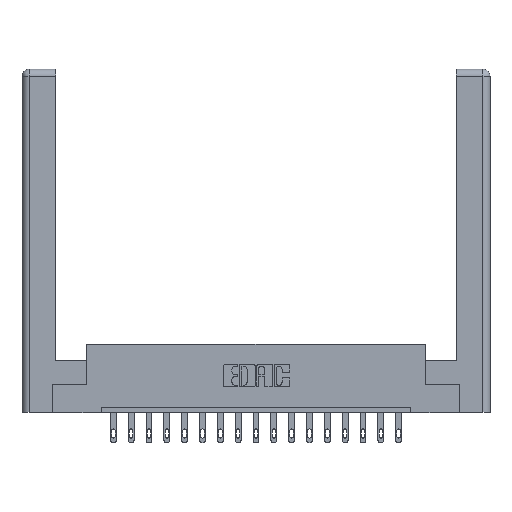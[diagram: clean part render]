
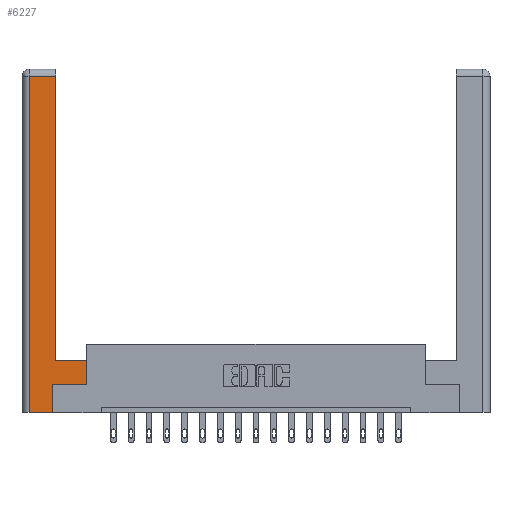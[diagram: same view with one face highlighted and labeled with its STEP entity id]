
A CAD part, top view. The second image highlights one B-rep face of the part: STEP entity #6227.
In plain terms, the highlighted planar face has unit normal (0, 0, 1).
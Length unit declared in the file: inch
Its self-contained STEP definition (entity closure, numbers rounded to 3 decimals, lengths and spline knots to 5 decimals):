
#343 = VECTOR ( 'NONE', #17578, 39.37008 ) ;
#776 = EDGE_CURVE ( 'NONE', #8534, #6111, #946, .T. ) ;
#886 = EDGE_CURVE ( 'NONE', #6111, #6273, #6243, .T. ) ;
#918 = VERTEX_POINT ( 'NONE', #2726 ) ;
#946 = LINE ( 'NONE', #7015, #6676 ) ;
#1485 = VERTEX_POINT ( 'NONE', #10920 ) ;
#1598 = DIRECTION ( 'NONE',  ( -1., 0., 0. ) ) ;
#2092 = ORIENTED_EDGE ( 'NONE', *, *, #776, .T. ) ;
#2726 = CARTESIAN_POINT ( 'NONE',  ( 0.295, 0.45, 0. ) ) ;
#2893 = DIRECTION ( 'NONE',  ( 1., 0., 0. ) ) ;
#3863 = VECTOR ( 'NONE', #5603, 39.37008 ) ;
#3894 = ORIENTED_EDGE ( 'NONE', *, *, #12068, .T. ) ;
#4445 = CARTESIAN_POINT ( 'NONE',  ( 0.0615, 0., 0. ) ) ;
#5168 = CARTESIAN_POINT ( 'NONE',  ( 0.0615, 2.94, 0. ) ) ;
#5186 = ORIENTED_EDGE ( 'NONE', *, *, #15403, .T. ) ;
#5531 = EDGE_CURVE ( 'NONE', #15382, #8534, #6439, .T. ) ;
#5540 = CARTESIAN_POINT ( 'NONE',  ( 0.295, 0.45, 0. ) ) ;
#5555 = CARTESIAN_POINT ( 'NONE',  ( 0.265, 0.245, 0. ) ) ;
#5603 = DIRECTION ( 'NONE',  ( 0., 1., 0. ) ) ;
#5663 = CARTESIAN_POINT ( 'NONE',  ( 0.0615, 0., 0. ) ) ;
#5736 = DIRECTION ( 'NONE',  ( 0., 0., -1. ) ) ;
#6111 = VERTEX_POINT ( 'NONE', #12034 ) ;
#6227 = ADVANCED_FACE ( 'NONE', ( #13368 ), #15789, .F. ) ;
#6243 = LINE ( 'NONE', #5555, #6922 ) ;
#6273 = VERTEX_POINT ( 'NONE', #8677 ) ;
#6439 = LINE ( 'NONE', #5663, #13622 ) ;
#6676 = VECTOR ( 'NONE', #2893, 39.37008 ) ;
#6922 = VECTOR ( 'NONE', #9826, 39.37008 ) ;
#7015 = CARTESIAN_POINT ( 'NONE',  ( 0.265, 0., 0. ) ) ;
#7219 = VERTEX_POINT ( 'NONE', #14689 ) ;
#7263 = CARTESIAN_POINT ( 'NONE',  ( 0., 0., 0. ) ) ;
#7483 = DIRECTION ( 'NONE',  ( -1., 0., 0. ) ) ;
#7595 = VECTOR ( 'NONE', #7483, 39.37008 ) ;
#7686 = EDGE_LOOP ( 'NONE', ( #10659, #12234, #14229, #2092, #7741, #5186, #14792, #3894 ) ) ;
#7741 = ORIENTED_EDGE ( 'NONE', *, *, #886, .T. ) ;
#8534 = VERTEX_POINT ( 'NONE', #4445 ) ;
#8553 = VERTEX_POINT ( 'NONE', #14397 ) ;
#8582 = EDGE_CURVE ( 'NONE', #918, #8553, #15037, .T. ) ;
#8664 = DIRECTION ( 'NONE',  ( 0., -1., 0. ) ) ;
#8677 = CARTESIAN_POINT ( 'NONE',  ( 0.265, 0.245, 0. ) ) ;
#9007 = EDGE_CURVE ( 'NONE', #1485, #7219, #12331, .T. ) ;
#9025 = CARTESIAN_POINT ( 'NONE',  ( 0.0615, 2.94, 0. ) ) ;
#9826 = DIRECTION ( 'NONE',  ( 0., 1., 0. ) ) ;
#9944 = DIRECTION ( 'NONE',  ( -1., 0., 0. ) ) ;
#9951 = CARTESIAN_POINT ( 'NONE',  ( 0.565, 0.45, 0. ) ) ;
#10659 = ORIENTED_EDGE ( 'NONE', *, *, #8582, .T. ) ;
#10674 = LINE ( 'NONE', #5540, #11349 ) ;
#10876 = DIRECTION ( 'NONE',  ( 1., 0., 0. ) ) ;
#10920 = CARTESIAN_POINT ( 'NONE',  ( 0.565, 0.245, 0. ) ) ;
#11349 = VECTOR ( 'NONE', #9944, 39.37008 ) ;
#11410 = LINE ( 'NONE', #9025, #7595 ) ;
#11773 = CARTESIAN_POINT ( 'NONE',  ( 0.295, 3., 0. ) ) ;
#12034 = CARTESIAN_POINT ( 'NONE',  ( 0.265, 0., 0. ) ) ;
#12068 = EDGE_CURVE ( 'NONE', #7219, #918, #10674, .T. ) ;
#12157 = AXIS2_PLACEMENT_3D ( 'NONE', #7263, #5736, #1598 ) ;
#12234 = ORIENTED_EDGE ( 'NONE', *, *, #17016, .T. ) ;
#12272 = CARTESIAN_POINT ( 'NONE',  ( 0.565, 0.245, 0. ) ) ;
#12331 = LINE ( 'NONE', #9951, #3863 ) ;
#13368 = FACE_OUTER_BOUND ( 'NONE', #7686, .T. ) ;
#13622 = VECTOR ( 'NONE', #8664, 39.37008 ) ;
#14229 = ORIENTED_EDGE ( 'NONE', *, *, #5531, .T. ) ;
#14397 = CARTESIAN_POINT ( 'NONE',  ( 0.295, 2.94, 0. ) ) ;
#14689 = CARTESIAN_POINT ( 'NONE',  ( 0.565, 0.45, 0. ) ) ;
#14792 = ORIENTED_EDGE ( 'NONE', *, *, #9007, .T. ) ;
#15037 = LINE ( 'NONE', #11773, #343 ) ;
#15275 = VECTOR ( 'NONE', #10876, 39.37008 ) ;
#15382 = VERTEX_POINT ( 'NONE', #5168 ) ;
#15403 = EDGE_CURVE ( 'NONE', #6273, #1485, #16827, .T. ) ;
#15789 = PLANE ( 'NONE',  #12157 ) ;
#16827 = LINE ( 'NONE', #12272, #15275 ) ;
#17016 = EDGE_CURVE ( 'NONE', #8553, #15382, #11410, .T. ) ;
#17578 = DIRECTION ( 'NONE',  ( 0., 1., 0. ) ) ;
